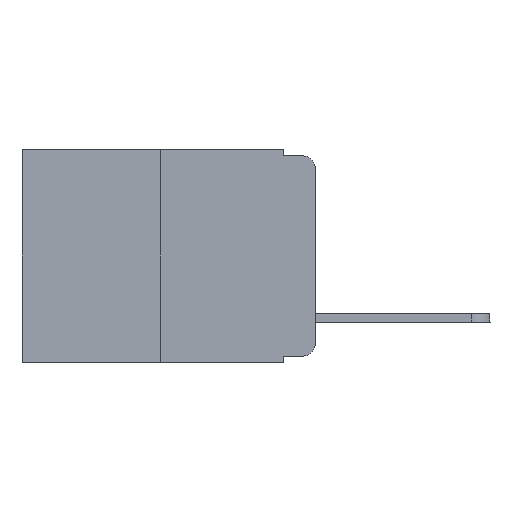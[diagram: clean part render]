
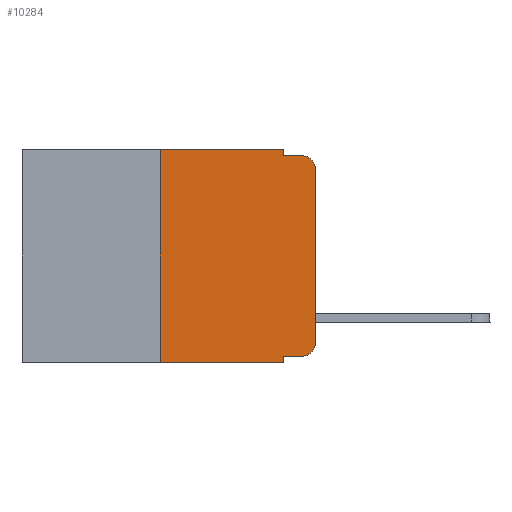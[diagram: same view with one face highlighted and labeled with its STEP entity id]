
A CAD part, left-side view. The second image highlights one B-rep face of the part: STEP entity #10284.
In plain terms, the highlighted planar face has unit normal (-1, 0, 0).
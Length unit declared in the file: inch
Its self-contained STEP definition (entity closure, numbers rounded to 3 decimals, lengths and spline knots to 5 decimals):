
#54 = DIRECTION ( 'NONE',  ( 0., -1., 0. ) ) ;
#336 = VECTOR ( 'NONE', #3000, 39.37008 ) ;
#526 = CARTESIAN_POINT ( 'NONE',  ( 0., 0.25, 0. ) ) ;
#925 = DIRECTION ( 'NONE',  ( 0., -1., 0. ) ) ;
#1063 = VECTOR ( 'NONE', #7019, 39.37008 ) ;
#1168 = CARTESIAN_POINT ( 'NONE',  ( 0., 0., 0. ) ) ;
#1393 = LINE ( 'NONE', #7762, #6393 ) ;
#1509 = DIRECTION ( 'NONE',  ( -1., 0., 0. ) ) ;
#1626 = VECTOR ( 'NONE', #7499, 39.37008 ) ;
#1641 = VERTEX_POINT ( 'NONE', #9273 ) ;
#1808 = LINE ( 'NONE', #1168, #9454 ) ;
#1910 = EDGE_CURVE ( 'NONE', #9959, #7298, #9504, .T. ) ;
#2183 = EDGE_CURVE ( 'NONE', #9959, #8708, #1393, .T. ) ;
#2370 = LINE ( 'NONE', #7986, #336 ) ;
#2680 = CARTESIAN_POINT ( 'NONE',  ( 0., 0.473, 0. ) ) ;
#3000 = DIRECTION ( 'NONE',  ( 0., -1., 0. ) ) ;
#3084 = EDGE_CURVE ( 'NONE', #6378, #4519, #7761, .T. ) ;
#3153 = CARTESIAN_POINT ( 'NONE',  ( 0., 0.473, 0. ) ) ;
#3202 = ORIENTED_EDGE ( 'NONE', *, *, #5819, .T. ) ;
#3623 = EDGE_CURVE ( 'NONE', #6274, #10470, #1808, .T. ) ;
#3796 = CARTESIAN_POINT ( 'NONE',  ( 0., 0.02, -0.333 ) ) ;
#3887 = CARTESIAN_POINT ( 'NONE',  ( 0., 0.051, -0.333 ) ) ;
#4229 = DIRECTION ( 'NONE',  ( -1., 0., 0. ) ) ;
#4307 = DIRECTION ( 'NONE',  ( 0., 0., 1. ) ) ;
#4391 = ORIENTED_EDGE ( 'NONE', *, *, #11185, .F. ) ;
#4519 = VERTEX_POINT ( 'NONE', #8398 ) ;
#4642 = ORIENTED_EDGE ( 'NONE', *, *, #11294, .F. ) ;
#4747 = CARTESIAN_POINT ( 'NONE',  ( 0., 0.051, 0. ) ) ;
#4926 = DIRECTION ( 'NONE',  ( 0., 0., -1. ) ) ;
#4947 = ORIENTED_EDGE ( 'NONE', *, *, #9929, .T. ) ;
#5011 = CARTESIAN_POINT ( 'NONE',  ( 0., 0.25, -0.343 ) ) ;
#5146 = DIRECTION ( 'NONE',  ( 0., 0., -1. ) ) ;
#5170 = AXIS2_PLACEMENT_3D ( 'NONE', #9276, #1509, #10146 ) ;
#5507 = EDGE_LOOP ( 'NONE', ( #7310, #3202, #4391, #10416, #4642, #10066, #4947, #10630, #10525, #10104 ) ) ;
#5629 = DIRECTION ( 'NONE',  ( 0., 0., -1. ) ) ;
#5774 = VECTOR ( 'NONE', #54, 39.37008 ) ;
#5819 = EDGE_CURVE ( 'NONE', #10470, #1641, #6202, .T. ) ;
#6004 = CARTESIAN_POINT ( 'NONE',  ( 0., 0., -0.313 ) ) ;
#6084 = LINE ( 'NONE', #12890, #5774 ) ;
#6121 = CIRCLE ( 'NONE', #8060, 0.02 ) ;
#6202 = CIRCLE ( 'NONE', #5170, 0.02 ) ;
#6274 = VERTEX_POINT ( 'NONE', #6004 ) ;
#6344 = CARTESIAN_POINT ( 'NONE',  ( 0., 0.051, 0. ) ) ;
#6378 = VERTEX_POINT ( 'NONE', #6344 ) ;
#6393 = VECTOR ( 'NONE', #4926, 39.37008 ) ;
#6543 = VECTOR ( 'NONE', #925, 39.37008 ) ;
#6944 = LINE ( 'NONE', #526, #1626 ) ;
#7019 = DIRECTION ( 'NONE',  ( 0., 0., -1. ) ) ;
#7180 = EDGE_CURVE ( 'NONE', #8747, #10288, #6944, .T. ) ;
#7298 = VERTEX_POINT ( 'NONE', #3796 ) ;
#7310 = ORIENTED_EDGE ( 'NONE', *, *, #3623, .T. ) ;
#7499 = DIRECTION ( 'NONE',  ( 0., 0., 1. ) ) ;
#7664 = PLANE ( 'NONE',  #9893 ) ;
#7761 = LINE ( 'NONE', #4747, #1063 ) ;
#7762 = CARTESIAN_POINT ( 'NONE',  ( 0., 0.051, 0. ) ) ;
#7800 = CARTESIAN_POINT ( 'NONE',  ( 0., 0., -0.03 ) ) ;
#7986 = CARTESIAN_POINT ( 'NONE',  ( 0., 0.473, -0.343 ) ) ;
#8060 = AXIS2_PLACEMENT_3D ( 'NONE', #11208, #4229, #5146 ) ;
#8398 = CARTESIAN_POINT ( 'NONE',  ( 0., 0.051, -0.01 ) ) ;
#8628 = DIRECTION ( 'NONE',  ( 1., 0., 0. ) ) ;
#8708 = VERTEX_POINT ( 'NONE', #9021 ) ;
#8726 = LINE ( 'NONE', #3153, #10759 ) ;
#8747 = VERTEX_POINT ( 'NONE', #5011 ) ;
#9021 = CARTESIAN_POINT ( 'NONE',  ( 0., 0.051, -0.343 ) ) ;
#9273 = CARTESIAN_POINT ( 'NONE',  ( 0., 0.02, -0.01 ) ) ;
#9276 = CARTESIAN_POINT ( 'NONE',  ( 0., 0.02, -0.03 ) ) ;
#9454 = VECTOR ( 'NONE', #4307, 39.37008 ) ;
#9504 = LINE ( 'NONE', #10750, #6543 ) ;
#9539 = CARTESIAN_POINT ( 'NONE',  ( 0., 0.25, 0. ) ) ;
#9893 = AXIS2_PLACEMENT_3D ( 'NONE', #2680, #8628, #5629 ) ;
#9929 = EDGE_CURVE ( 'NONE', #8747, #8708, #2370, .T. ) ;
#9959 = VERTEX_POINT ( 'NONE', #3887 ) ;
#10010 = EDGE_CURVE ( 'NONE', #7298, #6274, #6121, .T. ) ;
#10066 = ORIENTED_EDGE ( 'NONE', *, *, #7180, .F. ) ;
#10104 = ORIENTED_EDGE ( 'NONE', *, *, #10010, .T. ) ;
#10133 = DIRECTION ( 'NONE',  ( 0., -1., 0. ) ) ;
#10146 = DIRECTION ( 'NONE',  ( 0., 0., -1. ) ) ;
#10284 = ADVANCED_FACE ( 'NONE', ( #11720 ), #7664, .F. ) ;
#10288 = VERTEX_POINT ( 'NONE', #9539 ) ;
#10416 = ORIENTED_EDGE ( 'NONE', *, *, #3084, .F. ) ;
#10470 = VERTEX_POINT ( 'NONE', #7800 ) ;
#10525 = ORIENTED_EDGE ( 'NONE', *, *, #1910, .T. ) ;
#10630 = ORIENTED_EDGE ( 'NONE', *, *, #2183, .F. ) ;
#10750 = CARTESIAN_POINT ( 'NONE',  ( 0., 0.051, -0.333 ) ) ;
#10759 = VECTOR ( 'NONE', #10133, 39.37008 ) ;
#11185 = EDGE_CURVE ( 'NONE', #4519, #1641, #6084, .T. ) ;
#11208 = CARTESIAN_POINT ( 'NONE',  ( 0., 0.02, -0.313 ) ) ;
#11294 = EDGE_CURVE ( 'NONE', #10288, #6378, #8726, .T. ) ;
#11720 = FACE_OUTER_BOUND ( 'NONE', #5507, .T. ) ;
#12890 = CARTESIAN_POINT ( 'NONE',  ( 0., 0.051, -0.01 ) ) ;
